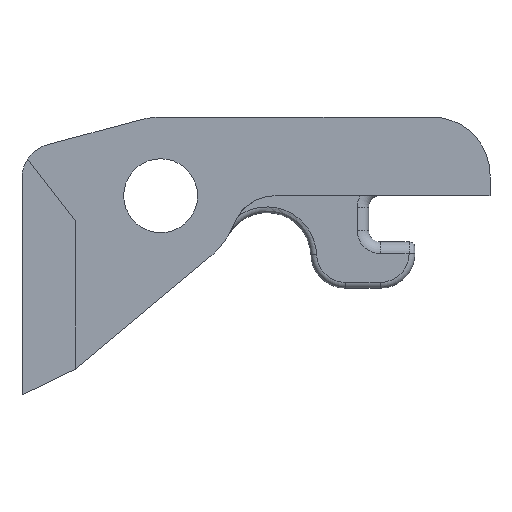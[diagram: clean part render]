
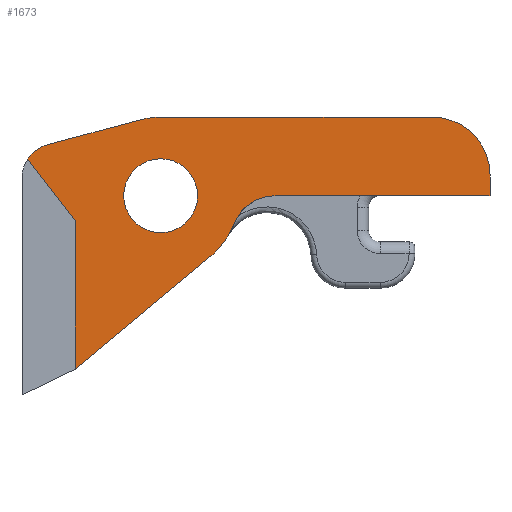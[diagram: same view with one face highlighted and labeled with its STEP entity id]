
A CAD part, left-side view. The second image highlights one B-rep face of the part: STEP entity #1673.
In plain terms, the highlighted planar face has unit normal (-1, 0, 0).
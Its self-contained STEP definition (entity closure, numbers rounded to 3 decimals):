
#84=CARTESIAN_POINT('',(-2.8,-23.5,6.8));
#85=VERTEX_POINT('',#84);
#92=CARTESIAN_POINT('',(-2.8,-28.5,1.8));
#93=VERTEX_POINT('',#92);
#94=CARTESIAN_POINT('',(-2.8,-23.5,1.8));
#95=DIRECTION('',(1.0,0.0,0.0));
#96=DIRECTION('',(0.0,-0.707,0.707));
#97=AXIS2_PLACEMENT_3D('',#94,#95,#96);
#98=CIRCLE('',#97,5.0);
#99=EDGE_CURVE('',#85,#93,#98,.T.);
#124=CARTESIAN_POINT('',(-2.8,0.0,6.8));
#125=VERTEX_POINT('',#124);
#132=CARTESIAN_POINT('',(-2.8,0.0,6.8));
#133=DIRECTION('',(0.0,-1.0,0.0));
#134=VECTOR('',#133,23.5);
#135=LINE('',#132,#134);
#136=EDGE_CURVE('',#125,#85,#135,.T.);
#1236=CARTESIAN_POINT('',(-2.8,11.503,3.176));
#1237=VERTEX_POINT('',#1236);
#1238=CARTESIAN_POINT('',(-2.8,9.776,4.42));
#1239=VERTEX_POINT('',#1238);
#1240=CARTESIAN_POINT('',(-2.8,9.,1.523));
#1241=DIRECTION('',(1.0,0.0,0.0));
#1242=DIRECTION('',(0.0,0.793,0.609));
#1243=AXIS2_PLACEMENT_3D('',#1240,#1241,#1242);
#1244=CIRCLE('',#1243,3.0);
#1245=EDGE_CURVE('',#1237,#1239,#1244,.T.);
#1359=CARTESIAN_POINT('',(-2.8,1.76,6.568));
#1360=VERTEX_POINT('',#1359);
#1361=CARTESIAN_POINT('',(-2.8,9.776,4.42));
#1362=DIRECTION('',(0.0,-0.966,0.259));
#1363=VECTOR('',#1362,8.299);
#1364=LINE('',#1361,#1363);
#1365=EDGE_CURVE('',#1239,#1360,#1364,.T.);
#1462=CARTESIAN_POINT('',(-2.8,-28.5,0.));
#1463=VERTEX_POINT('',#1462);
#1470=CARTESIAN_POINT('',(-2.8,-9.895,0.));
#1471=VERTEX_POINT('',#1470);
#1472=CARTESIAN_POINT('',(-2.8,-28.5,0.));
#1473=DIRECTION('',(0.0,1.0,0.0));
#1474=VECTOR('',#1473,18.605);
#1475=LINE('',#1472,#1474);
#1476=EDGE_CURVE('',#1463,#1471,#1475,.T.);
#1512=CARTESIAN_POINT('',(-2.8,-6.348,-2.438));
#1513=VERTEX_POINT('',#1512);
#1514=CARTESIAN_POINT('',(-2.8,-9.895,-3.8));
#1515=DIRECTION('',(-1.0,0.0,0.0));
#1516=DIRECTION('',(0.0,0.566,0.824));
#1517=AXIS2_PLACEMENT_3D('',#1514,#1515,#1516);
#1518=CIRCLE('',#1517,3.8);
#1519=EDGE_CURVE('',#1471,#1513,#1518,.T.);
#1536=CARTESIAN_POINT('',(-2.8,3.2,0.));
#1537=VERTEX_POINT('',#1536);
#1538=CARTESIAN_POINT('',(-2.8,0.0,0.0));
#1539=DIRECTION('',(1.0,0.0,0.0));
#1540=DIRECTION('',(0.0,-1.0,0.0));
#1541=AXIS2_PLACEMENT_3D('',#1538,#1539,#1540);
#1542=CIRCLE('',#1541,3.2);
#1543=EDGE_CURVE('',#1537,#1537,#1542,.T.);
#1557=CARTESIAN_POINT('',(-2.8,-28.5,1.8));
#1558=DIRECTION('',(0.0,0.0,-1.0));
#1559=VECTOR('',#1558,1.8);
#1560=LINE('',#1557,#1559);
#1561=EDGE_CURVE('',#93,#1463,#1560,.T.);
#1574=CARTESIAN_POINT('',(-2.8,-4.348,-5.228));
#1575=VERTEX_POINT('',#1574);
#1576=CARTESIAN_POINT('',(-2.8,0.0,0.0));
#1577=DIRECTION('',(1.0,0.0,0.0));
#1578=DIRECTION('',(0.0,1.0,0.0));
#1579=AXIS2_PLACEMENT_3D('',#1576,#1577,#1578);
#1580=CIRCLE('',#1579,6.8);
#1581=EDGE_CURVE('',#1513,#1575,#1580,.T.);
#1605=CARTESIAN_POINT('',(-2.8,0.0,0.0));
#1606=DIRECTION('',(1.0,0.0,0.0));
#1607=DIRECTION('',(0.0,1.0,0.0));
#1608=AXIS2_PLACEMENT_3D('',#1605,#1606,#1607);
#1609=CIRCLE('',#1608,6.8);
#1610=EDGE_CURVE('',#1360,#125,#1609,.T.);
#1622=CARTESIAN_POINT('',(-2.8,7.4,-15.0));
#1623=VERTEX_POINT('',#1622);
#1624=CARTESIAN_POINT('',(-2.8,-4.348,-5.228));
#1625=DIRECTION('',(0.0,0.769,-0.639));
#1626=VECTOR('',#1625,15.281);
#1627=LINE('',#1624,#1626);
#1628=EDGE_CURVE('',#1575,#1623,#1627,.T.);
#1639=CARTESIAN_POINT('',(-2.8,8.94,1.584));
#1640=DIRECTION('',(1.0,0.0,0.0));
#1641=DIRECTION('',(0.0,0.0,-1.0));
#1642=AXIS2_PLACEMENT_3D('',#1639,#1640,#1641);
#1643=PLANE('',#1642);
#1644=ORIENTED_EDGE('',*,*,#99,.F.);
#1645=ORIENTED_EDGE('',*,*,#136,.F.);
#1646=ORIENTED_EDGE('',*,*,#1610,.F.);
#1647=ORIENTED_EDGE('',*,*,#1365,.F.);
#1648=ORIENTED_EDGE('',*,*,#1245,.F.);
#1649=CARTESIAN_POINT('',(-2.8,7.4,-2.176));
#1650=VERTEX_POINT('',#1649);
#1651=CARTESIAN_POINT('',(-2.8,7.4,-2.176));
#1652=DIRECTION('',(0.0,0.608,0.794));
#1653=VECTOR('',#1652,6.744);
#1654=LINE('',#1651,#1653);
#1655=EDGE_CURVE('',#1650,#1237,#1654,.T.);
#1656=ORIENTED_EDGE('',*,*,#1655,.F.);
#1657=CARTESIAN_POINT('',(-2.8,7.4,-15.0));
#1658=DIRECTION('',(0.0,0.0,1.0));
#1659=VECTOR('',#1658,12.824);
#1660=LINE('',#1657,#1659);
#1661=EDGE_CURVE('',#1623,#1650,#1660,.T.);
#1662=ORIENTED_EDGE('',*,*,#1661,.F.);
#1663=ORIENTED_EDGE('',*,*,#1628,.F.);
#1664=ORIENTED_EDGE('',*,*,#1581,.F.);
#1665=ORIENTED_EDGE('',*,*,#1519,.F.);
#1666=ORIENTED_EDGE('',*,*,#1476,.F.);
#1667=ORIENTED_EDGE('',*,*,#1561,.F.);
#1668=EDGE_LOOP('',(#1644,#1645,#1646,#1647,#1648,#1656,#1662,#1663,#1664,#1665,#1666,#1667));
#1669=FACE_OUTER_BOUND('',#1668,.T.);
#1670=ORIENTED_EDGE('',*,*,#1543,.T.);
#1671=EDGE_LOOP('',(#1670));
#1672=FACE_BOUND('',#1671,.T.);
#1673=ADVANCED_FACE('',(#1669,#1672),#1643,.F.);
